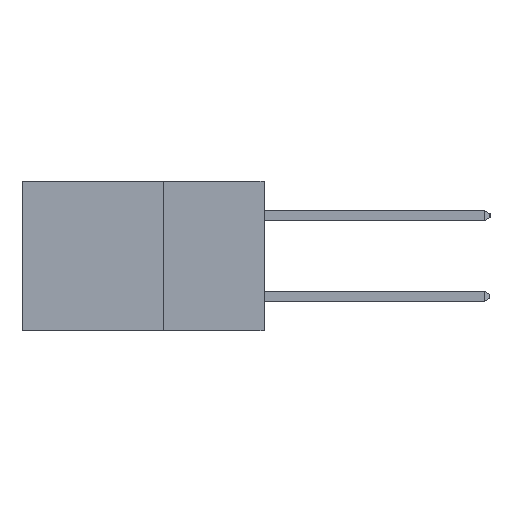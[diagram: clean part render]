
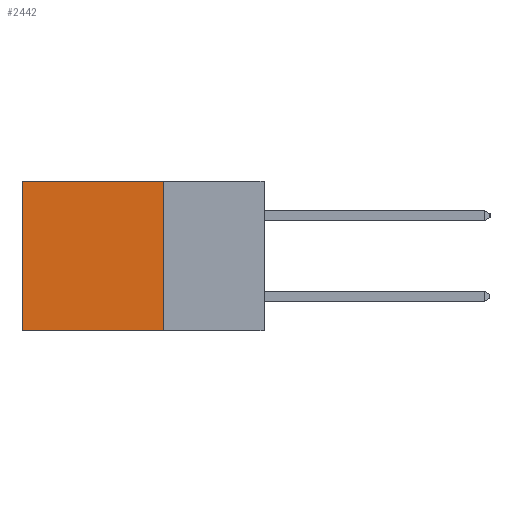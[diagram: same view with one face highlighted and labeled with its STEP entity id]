
A CAD part, left-side view. The second image highlights one B-rep face of the part: STEP entity #2442.
In plain terms, the highlighted planar face has unit normal (-1, 0, 0).
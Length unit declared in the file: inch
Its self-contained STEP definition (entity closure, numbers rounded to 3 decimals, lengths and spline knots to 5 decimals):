
#459 = CARTESIAN_POINT ( 'NONE',  ( 0.298, 0.25, 0. ) ) ;
#1236 = VERTEX_POINT ( 'NONE', #16563 ) ;
#1405 = CARTESIAN_POINT ( 'NONE',  ( 0.298, 0.25, 0. ) ) ;
#1992 = EDGE_CURVE ( 'NONE', #1236, #9899, #7154, .T. ) ;
#2046 = ORIENTED_EDGE ( 'NONE', *, *, #17613, .T. ) ;
#2281 = AXIS2_PLACEMENT_3D ( 'NONE', #8304, #6500, #10791 ) ;
#2442 = ADVANCED_FACE ( 'NONE', ( #14289 ), #9993, .F. ) ;
#3931 = ORIENTED_EDGE ( 'NONE', *, *, #1992, .F. ) ;
#4302 = DIRECTION ( 'NONE',  ( 0., 1., 0. ) ) ;
#4817 = ORIENTED_EDGE ( 'NONE', *, *, #7362, .T. ) ;
#5007 = VERTEX_POINT ( 'NONE', #12879 ) ;
#5465 = VERTEX_POINT ( 'NONE', #459 ) ;
#5514 = DIRECTION ( 'NONE',  ( 0., 0., -1. ) ) ;
#5779 = VECTOR ( 'NONE', #5514, 39.37008 ) ;
#6116 = LINE ( 'NONE', #6738, #10221 ) ;
#6496 = VECTOR ( 'NONE', #13883, 39.37008 ) ;
#6500 = DIRECTION ( 'NONE',  ( 1., 0., 0. ) ) ;
#6738 = CARTESIAN_POINT ( 'NONE',  ( 0.298, 0.6, 0. ) ) ;
#6857 = CARTESIAN_POINT ( 'NONE',  ( 0.298, 0.25, 0. ) ) ;
#7154 = LINE ( 'NONE', #12967, #13892 ) ;
#7362 = EDGE_CURVE ( 'NONE', #5007, #9899, #6116, .T. ) ;
#8304 = CARTESIAN_POINT ( 'NONE',  ( 0.298, 0.25, 0. ) ) ;
#9449 = LINE ( 'NONE', #6857, #5779 ) ;
#9899 = VERTEX_POINT ( 'NONE', #16548 ) ;
#9993 = PLANE ( 'NONE',  #2281 ) ;
#10045 = ORIENTED_EDGE ( 'NONE', *, *, #13876, .F. ) ;
#10221 = VECTOR ( 'NONE', #16068, 39.37008 ) ;
#10791 = DIRECTION ( 'NONE',  ( 0., 0., -1. ) ) ;
#12879 = CARTESIAN_POINT ( 'NONE',  ( 0.298, 0.6, 0. ) ) ;
#12967 = CARTESIAN_POINT ( 'NONE',  ( 0.298, 0.25, -0.37 ) ) ;
#13876 = EDGE_CURVE ( 'NONE', #5465, #1236, #9449, .T. ) ;
#13883 = DIRECTION ( 'NONE',  ( 0., 1., 0. ) ) ;
#13892 = VECTOR ( 'NONE', #4302, 39.37008 ) ;
#14289 = FACE_OUTER_BOUND ( 'NONE', #14948, .T. ) ;
#14948 = EDGE_LOOP ( 'NONE', ( #4817, #3931, #10045, #2046 ) ) ;
#16068 = DIRECTION ( 'NONE',  ( 0., 0., -1. ) ) ;
#16548 = CARTESIAN_POINT ( 'NONE',  ( 0.298, 0.6, -0.37 ) ) ;
#16563 = CARTESIAN_POINT ( 'NONE',  ( 0.298, 0.25, -0.37 ) ) ;
#17496 = LINE ( 'NONE', #1405, #6496 ) ;
#17613 = EDGE_CURVE ( 'NONE', #5465, #5007, #17496, .T. ) ;
